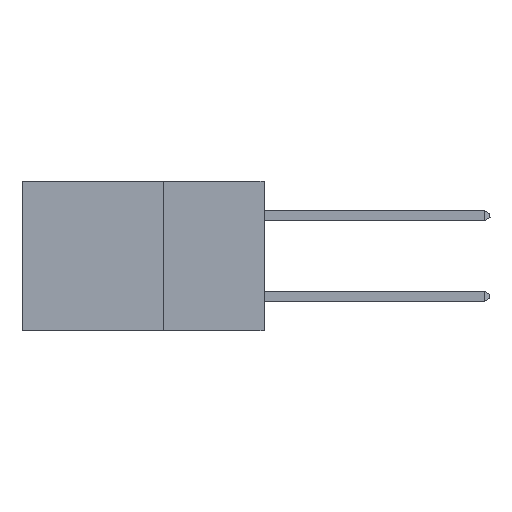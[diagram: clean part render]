
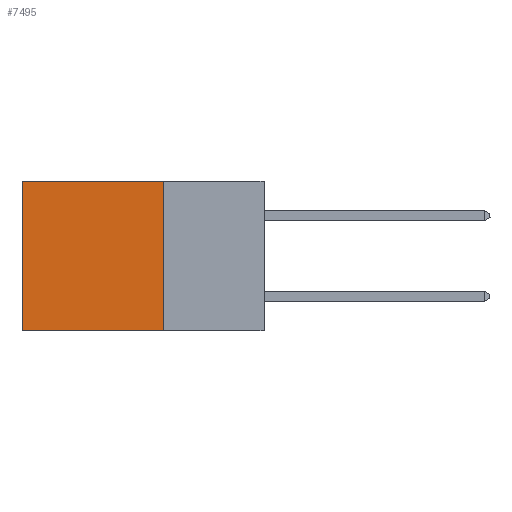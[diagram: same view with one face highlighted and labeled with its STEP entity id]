
A CAD part, left-side view. The second image highlights one B-rep face of the part: STEP entity #7495.
In plain terms, the highlighted planar face has unit normal (-1, 0, 0).
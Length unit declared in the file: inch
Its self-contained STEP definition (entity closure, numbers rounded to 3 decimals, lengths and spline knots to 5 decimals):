
#276 = FACE_OUTER_BOUND ( 'NONE', #17248, .T. ) ;
#872 = CARTESIAN_POINT ( 'NONE',  ( 0.298, 0.25, 0. ) ) ;
#885 = LINE ( 'NONE', #16074, #8889 ) ;
#1008 = DIRECTION ( 'NONE',  ( 0., 0., -1. ) ) ;
#1032 = CARTESIAN_POINT ( 'NONE',  ( 0.298, 0.25, 0. ) ) ;
#1082 = DIRECTION ( 'NONE',  ( 1., 0., 0. ) ) ;
#2788 = VERTEX_POINT ( 'NONE', #15584 ) ;
#2837 = ORIENTED_EDGE ( 'NONE', *, *, #16926, .F. ) ;
#3280 = VERTEX_POINT ( 'NONE', #7323 ) ;
#3288 = ORIENTED_EDGE ( 'NONE', *, *, #17806, .T. ) ;
#4663 = VERTEX_POINT ( 'NONE', #9668 ) ;
#5237 = LINE ( 'NONE', #16039, #5699 ) ;
#5699 = VECTOR ( 'NONE', #18868, 39.37008 ) ;
#6180 = CARTESIAN_POINT ( 'NONE',  ( 0.298, 0.25, -0.37 ) ) ;
#6692 = PLANE ( 'NONE',  #9930 ) ;
#7323 = CARTESIAN_POINT ( 'NONE',  ( 0.298, 0.25, 0. ) ) ;
#7495 = ADVANCED_FACE ( 'NONE', ( #276 ), #6692, .F. ) ;
#7870 = EDGE_CURVE ( 'NONE', #3280, #4663, #10081, .T. ) ;
#8298 = ORIENTED_EDGE ( 'NONE', *, *, #18631, .T. ) ;
#8889 = VECTOR ( 'NONE', #17587, 39.37008 ) ;
#9668 = CARTESIAN_POINT ( 'NONE',  ( 0.298, 0.25, -0.37 ) ) ;
#9868 = VECTOR ( 'NONE', #11108, 39.37008 ) ;
#9930 = AXIS2_PLACEMENT_3D ( 'NONE', #872, #1082, #1008 ) ;
#10081 = LINE ( 'NONE', #1032, #9868 ) ;
#10918 = DIRECTION ( 'NONE',  ( 0., 1., 0. ) ) ;
#11108 = DIRECTION ( 'NONE',  ( 0., 0., -1. ) ) ;
#13620 = CARTESIAN_POINT ( 'NONE',  ( 0.298, 0.6, -0.37 ) ) ;
#15023 = VERTEX_POINT ( 'NONE', #13620 ) ;
#15335 = LINE ( 'NONE', #6180, #17214 ) ;
#15584 = CARTESIAN_POINT ( 'NONE',  ( 0.298, 0.6, 0. ) ) ;
#16039 = CARTESIAN_POINT ( 'NONE',  ( 0.298, 0.6, 0. ) ) ;
#16074 = CARTESIAN_POINT ( 'NONE',  ( 0.298, 0.25, 0. ) ) ;
#16926 = EDGE_CURVE ( 'NONE', #4663, #15023, #15335, .T. ) ;
#17214 = VECTOR ( 'NONE', #10918, 39.37008 ) ;
#17248 = EDGE_LOOP ( 'NONE', ( #3288, #2837, #18103, #8298 ) ) ;
#17587 = DIRECTION ( 'NONE',  ( 0., 1., 0. ) ) ;
#17806 = EDGE_CURVE ( 'NONE', #2788, #15023, #5237, .T. ) ;
#18103 = ORIENTED_EDGE ( 'NONE', *, *, #7870, .F. ) ;
#18631 = EDGE_CURVE ( 'NONE', #3280, #2788, #885, .T. ) ;
#18868 = DIRECTION ( 'NONE',  ( 0., 0., -1. ) ) ;
